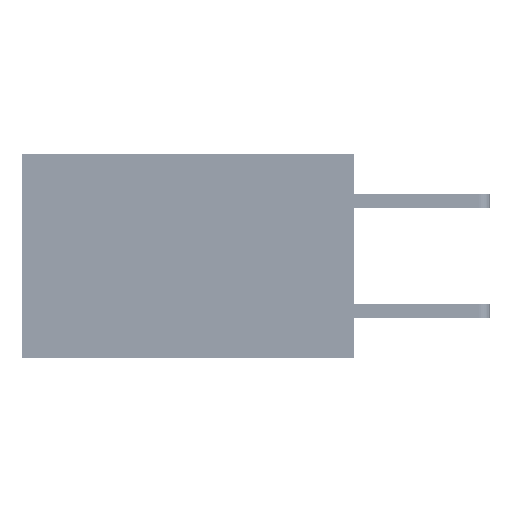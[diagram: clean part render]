
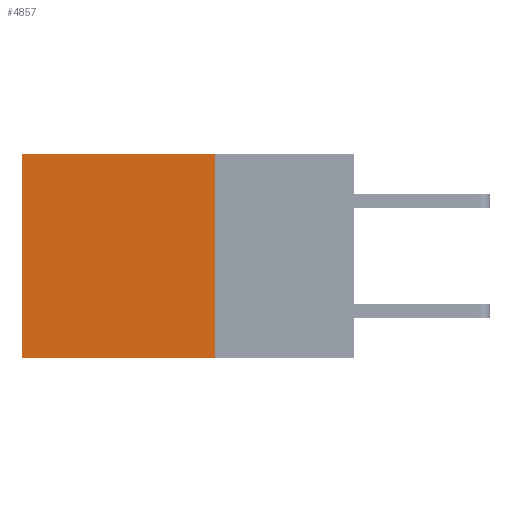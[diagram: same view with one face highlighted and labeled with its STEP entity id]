
A CAD part, left-side view. The second image highlights one B-rep face of the part: STEP entity #4857.
In plain terms, the highlighted planar face has unit normal (-1, 0, 0).
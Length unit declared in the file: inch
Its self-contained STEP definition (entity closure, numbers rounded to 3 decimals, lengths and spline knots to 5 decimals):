
#2909 = VECTOR ( 'NONE', #20073, 39.37008 ) ;
#4857 = ADVANCED_FACE ( 'NONE', ( #50942 ), #15206, .F. ) ;
#5279 = LINE ( 'NONE', #25622, #24649 ) ;
#7863 = CARTESIAN_POINT ( 'NONE',  ( 0.2875, 0.25, 0. ) ) ;
#10036 = CARTESIAN_POINT ( 'NONE',  ( 0.2875, 0.25, 0. ) ) ;
#12577 = ORIENTED_EDGE ( 'NONE', *, *, #21291, .T. ) ;
#13923 = ORIENTED_EDGE ( 'NONE', *, *, #19013, .F. ) ;
#15206 = PLANE ( 'NONE',  #38170 ) ;
#19013 = EDGE_CURVE ( 'NONE', #50472, #20254, #19811, .T. ) ;
#19525 = CARTESIAN_POINT ( 'NONE',  ( 0.2875, 0.25, -0.37 ) ) ;
#19654 = DIRECTION ( 'NONE',  ( 0., 1., 0. ) ) ;
#19811 = LINE ( 'NONE', #39898, #2909 ) ;
#20073 = DIRECTION ( 'NONE',  ( 0., 1., 0. ) ) ;
#20254 = VERTEX_POINT ( 'NONE', #28186 ) ;
#20860 = VECTOR ( 'NONE', #19654, 39.37008 ) ;
#21291 = EDGE_CURVE ( 'NONE', #47747, #20254, #5279, .T. ) ;
#22015 = ORIENTED_EDGE ( 'NONE', *, *, #47206, .T. ) ;
#23571 = CARTESIAN_POINT ( 'NONE',  ( 0.2875, 0.25, 0. ) ) ;
#24649 = VECTOR ( 'NONE', #25352, 39.37008 ) ;
#25352 = DIRECTION ( 'NONE',  ( 0., 0., -1. ) ) ;
#25622 = CARTESIAN_POINT ( 'NONE',  ( 0.2875, 0.6, 0. ) ) ;
#27456 = CARTESIAN_POINT ( 'NONE',  ( 0.2875, 0.25, 0. ) ) ;
#27487 = LINE ( 'NONE', #23571, #20860 ) ;
#28186 = CARTESIAN_POINT ( 'NONE',  ( 0.2875, 0.6, -0.37 ) ) ;
#33391 = EDGE_LOOP ( 'NONE', ( #12577, #13923, #47160, #22015 ) ) ;
#35256 = DIRECTION ( 'NONE',  ( 0., 0., -1. ) ) ;
#36720 = VECTOR ( 'NONE', #35256, 39.37008 ) ;
#38170 = AXIS2_PLACEMENT_3D ( 'NONE', #27456, #43115, #50163 ) ;
#39685 = LINE ( 'NONE', #7863, #36720 ) ;
#39898 = CARTESIAN_POINT ( 'NONE',  ( 0.2875, 0.25, -0.37 ) ) ;
#40191 = CARTESIAN_POINT ( 'NONE',  ( 0.2875, 0.6, 0. ) ) ;
#43115 = DIRECTION ( 'NONE',  ( 1., 0., 0. ) ) ;
#46968 = VERTEX_POINT ( 'NONE', #10036 ) ;
#47160 = ORIENTED_EDGE ( 'NONE', *, *, #47652, .F. ) ;
#47206 = EDGE_CURVE ( 'NONE', #46968, #47747, #27487, .T. ) ;
#47652 = EDGE_CURVE ( 'NONE', #46968, #50472, #39685, .T. ) ;
#47747 = VERTEX_POINT ( 'NONE', #40191 ) ;
#50163 = DIRECTION ( 'NONE',  ( 0., 0., -1. ) ) ;
#50472 = VERTEX_POINT ( 'NONE', #19525 ) ;
#50942 = FACE_OUTER_BOUND ( 'NONE', #33391, .T. ) ;
